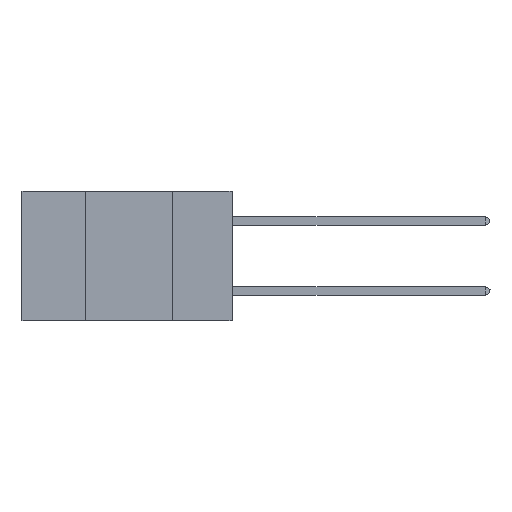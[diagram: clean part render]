
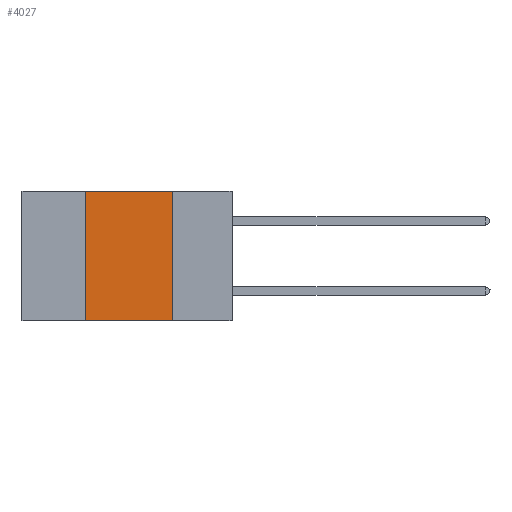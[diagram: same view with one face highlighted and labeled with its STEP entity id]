
A CAD part, left-side view. The second image highlights one B-rep face of the part: STEP entity #4027.
In plain terms, the highlighted planar face has unit normal (-1, 0, 0).
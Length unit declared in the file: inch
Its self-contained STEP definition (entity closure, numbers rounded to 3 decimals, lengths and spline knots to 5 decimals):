
#264 = LINE ( 'NONE', #14614, #14690 ) ;
#1416 = VERTEX_POINT ( 'NONE', #4319 ) ;
#1640 = FACE_OUTER_BOUND ( 'NONE', #20117, .T. ) ;
#3575 = DIRECTION ( 'NONE',  ( 0., 0., -1. ) ) ;
#4027 = ADVANCED_FACE ( 'NONE', ( #1640 ), #26544, .F. ) ;
#4118 = EDGE_CURVE ( 'NONE', #11091, #1416, #264, .T. ) ;
#4319 = CARTESIAN_POINT ( 'NONE',  ( 0., 0.17, -0.37 ) ) ;
#5330 = CARTESIAN_POINT ( 'NONE',  ( 0., 0.6, -0.37 ) ) ;
#5350 = ORIENTED_EDGE ( 'NONE', *, *, #20237, .F. ) ;
#6572 = VERTEX_POINT ( 'NONE', #11545 ) ;
#6712 = LINE ( 'NONE', #5330, #20822 ) ;
#7797 = VECTOR ( 'NONE', #10861, 39.37008 ) ;
#8942 = EDGE_CURVE ( 'NONE', #15029, #6572, #11007, .T. ) ;
#9047 = AXIS2_PLACEMENT_3D ( 'NONE', #14197, #18480, #3575 ) ;
#10861 = DIRECTION ( 'NONE',  ( 0., 0., 1. ) ) ;
#11007 = LINE ( 'NONE', #17327, #7797 ) ;
#11091 = VERTEX_POINT ( 'NONE', #18448 ) ;
#11545 = CARTESIAN_POINT ( 'NONE',  ( 0., 0.42, 0. ) ) ;
#13803 = ORIENTED_EDGE ( 'NONE', *, *, #4118, .F. ) ;
#14125 = ORIENTED_EDGE ( 'NONE', *, *, #17071, .T. ) ;
#14197 = CARTESIAN_POINT ( 'NONE',  ( 0., 0.6, 0. ) ) ;
#14614 = CARTESIAN_POINT ( 'NONE',  ( 0., 0.17, 0. ) ) ;
#14690 = VECTOR ( 'NONE', #15533, 39.37008 ) ;
#15029 = VERTEX_POINT ( 'NONE', #23991 ) ;
#15533 = DIRECTION ( 'NONE',  ( 0., 0., -1. ) ) ;
#16896 = ORIENTED_EDGE ( 'NONE', *, *, #8942, .F. ) ;
#17071 = EDGE_CURVE ( 'NONE', #15029, #1416, #6712, .T. ) ;
#17131 = CARTESIAN_POINT ( 'NONE',  ( 0., 0.6, 0. ) ) ;
#17327 = CARTESIAN_POINT ( 'NONE',  ( 0., 0.42, 0. ) ) ;
#18448 = CARTESIAN_POINT ( 'NONE',  ( 0., 0.17, 0. ) ) ;
#18480 = DIRECTION ( 'NONE',  ( 1., 0., 0. ) ) ;
#18938 = LINE ( 'NONE', #17131, #19217 ) ;
#19217 = VECTOR ( 'NONE', #22886, 39.37008 ) ;
#20117 = EDGE_LOOP ( 'NONE', ( #13803, #5350, #16896, #14125 ) ) ;
#20237 = EDGE_CURVE ( 'NONE', #6572, #11091, #18938, .T. ) ;
#20822 = VECTOR ( 'NONE', #24212, 39.37008 ) ;
#22886 = DIRECTION ( 'NONE',  ( 0., -1., 0. ) ) ;
#23991 = CARTESIAN_POINT ( 'NONE',  ( 0., 0.42, -0.37 ) ) ;
#24212 = DIRECTION ( 'NONE',  ( 0., -1., 0. ) ) ;
#26544 = PLANE ( 'NONE',  #9047 ) ;
